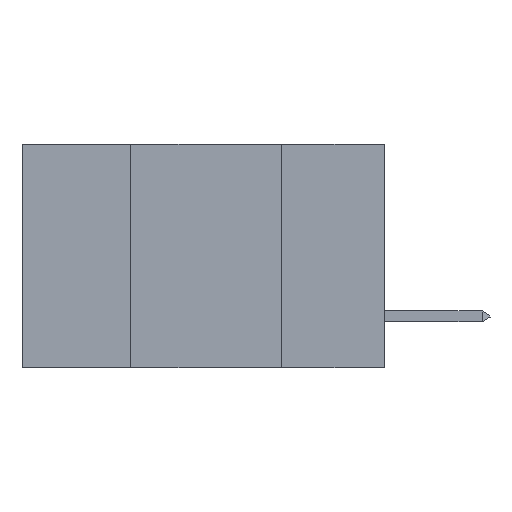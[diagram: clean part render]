
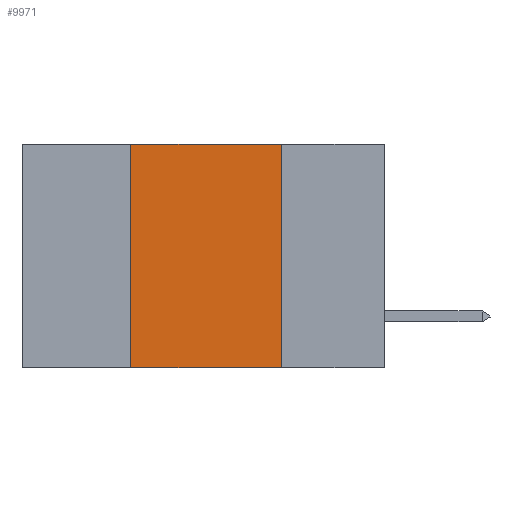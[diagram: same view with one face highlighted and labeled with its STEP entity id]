
A CAD part, left-side view. The second image highlights one B-rep face of the part: STEP entity #9971.
In plain terms, the highlighted planar face has unit normal (-1, 0, 0).
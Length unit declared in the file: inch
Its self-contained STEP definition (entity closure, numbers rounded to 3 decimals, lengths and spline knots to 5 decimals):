
#3223 = ORIENTED_EDGE ( 'NONE', *, *, #4677, .F. ) ;
#3938 = DIRECTION ( 'NONE',  ( 0., -1., 0. ) ) ;
#4004 = LINE ( 'NONE', #22857, #28025 ) ;
#4352 = ORIENTED_EDGE ( 'NONE', *, *, #4498, .F. ) ;
#4498 = EDGE_CURVE ( 'NONE', #9484, #14338, #10238, .T. ) ;
#4637 = ORIENTED_EDGE ( 'NONE', *, *, #39213, .T. ) ;
#4677 = EDGE_CURVE ( 'NONE', #14338, #22702, #37170, .T. ) ;
#4844 = FACE_OUTER_BOUND ( 'NONE', #15239, .T. ) ;
#5035 = EDGE_CURVE ( 'NONE', #22702, #17354, #9708, .T. ) ;
#9484 = VERTEX_POINT ( 'NONE', #32466 ) ;
#9708 = LINE ( 'NONE', #24299, #26541 ) ;
#9971 = ADVANCED_FACE ( 'NONE', ( #4844 ), #31565, .F. ) ;
#10238 = LINE ( 'NONE', #34863, #21262 ) ;
#10376 = CARTESIAN_POINT ( 'NONE',  ( 0., 0.17, -0.37 ) ) ;
#10467 = ORIENTED_EDGE ( 'NONE', *, *, #5035, .F. ) ;
#12391 = CARTESIAN_POINT ( 'NONE',  ( 0., 0.6, 0. ) ) ;
#13079 = VECTOR ( 'NONE', #3938, 39.37008 ) ;
#14338 = VERTEX_POINT ( 'NONE', #37712 ) ;
#14619 = CARTESIAN_POINT ( 'NONE',  ( 0., 0.17, 0. ) ) ;
#15239 = EDGE_LOOP ( 'NONE', ( #10467, #3223, #4352, #4637 ) ) ;
#17354 = VERTEX_POINT ( 'NONE', #10376 ) ;
#21078 = DIRECTION ( 'NONE',  ( 0., 0., -1. ) ) ;
#21165 = DIRECTION ( 'NONE',  ( 0., 0., -1. ) ) ;
#21262 = VECTOR ( 'NONE', #28924, 39.37008 ) ;
#22702 = VERTEX_POINT ( 'NONE', #14619 ) ;
#22857 = CARTESIAN_POINT ( 'NONE',  ( 0., 0.6, -0.37 ) ) ;
#24299 = CARTESIAN_POINT ( 'NONE',  ( 0., 0.17, 0. ) ) ;
#26541 = VECTOR ( 'NONE', #21165, 39.37008 ) ;
#28025 = VECTOR ( 'NONE', #38242, 39.37008 ) ;
#28924 = DIRECTION ( 'NONE',  ( 0., 0., 1. ) ) ;
#30383 = AXIS2_PLACEMENT_3D ( 'NONE', #35262, #39563, #21078 ) ;
#31565 = PLANE ( 'NONE',  #30383 ) ;
#32466 = CARTESIAN_POINT ( 'NONE',  ( 0., 0.42, -0.37 ) ) ;
#34863 = CARTESIAN_POINT ( 'NONE',  ( 0., 0.42, 0. ) ) ;
#35262 = CARTESIAN_POINT ( 'NONE',  ( 0., 0.6, 0. ) ) ;
#37170 = LINE ( 'NONE', #12391, #13079 ) ;
#37712 = CARTESIAN_POINT ( 'NONE',  ( 0., 0.42, 0. ) ) ;
#38242 = DIRECTION ( 'NONE',  ( 0., -1., 0. ) ) ;
#39213 = EDGE_CURVE ( 'NONE', #9484, #17354, #4004, .T. ) ;
#39563 = DIRECTION ( 'NONE',  ( 1., 0., 0. ) ) ;
